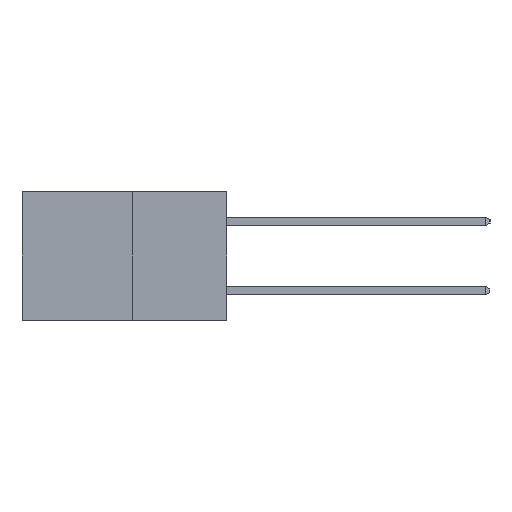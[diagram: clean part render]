
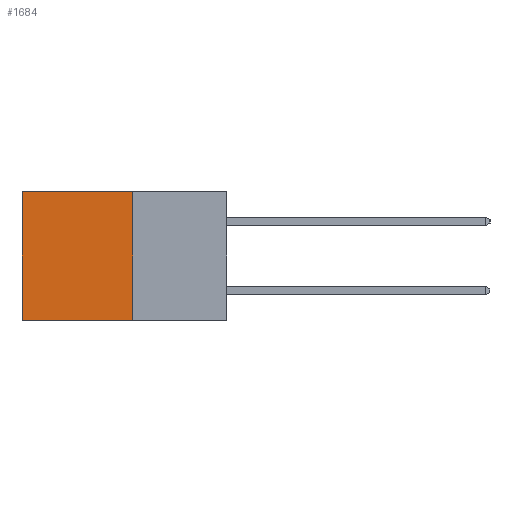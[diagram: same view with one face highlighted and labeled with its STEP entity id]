
A CAD part, left-side view. The second image highlights one B-rep face of the part: STEP entity #1684.
In plain terms, the highlighted planar face has unit normal (-1, 0, 0).
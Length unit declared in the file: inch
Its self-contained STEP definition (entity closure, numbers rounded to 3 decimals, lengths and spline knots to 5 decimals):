
#483 = VECTOR ( 'NONE', #691, 39.37008 ) ;
#499 = VERTEX_POINT ( 'NONE', #6705 ) ;
#691 = DIRECTION ( 'NONE',  ( 0., 1., 0. ) ) ;
#1018 = CARTESIAN_POINT ( 'NONE',  ( 0.277, 0.27, 0. ) ) ;
#1332 = EDGE_CURVE ( 'NONE', #8861, #1593, #4033, .T. ) ;
#1593 = VERTEX_POINT ( 'NONE', #8602 ) ;
#1684 = ADVANCED_FACE ( 'NONE', ( #2966 ), #6018, .F. ) ;
#2066 = VECTOR ( 'NONE', #5697, 39.37008 ) ;
#2381 = VECTOR ( 'NONE', #3738, 39.37008 ) ;
#2390 = LINE ( 'NONE', #8132, #8257 ) ;
#2966 = FACE_OUTER_BOUND ( 'NONE', #6873, .T. ) ;
#3132 = EDGE_CURVE ( 'NONE', #8741, #8861, #8332, .T. ) ;
#3738 = DIRECTION ( 'NONE',  ( 0., 0., -1. ) ) ;
#4033 = LINE ( 'NONE', #6846, #2066 ) ;
#4319 = CARTESIAN_POINT ( 'NONE',  ( 0.277, 0.27, -0.37 ) ) ;
#4415 = AXIS2_PLACEMENT_3D ( 'NONE', #4319, #5920, #5888 ) ;
#4494 = DIRECTION ( 'NONE',  ( 0., 1., 0. ) ) ;
#4719 = CARTESIAN_POINT ( 'NONE',  ( 0.277, 0.59, 0. ) ) ;
#5697 = DIRECTION ( 'NONE',  ( 0., 0., -1. ) ) ;
#5743 = ORIENTED_EDGE ( 'NONE', *, *, #3132, .T. ) ;
#5785 = ORIENTED_EDGE ( 'NONE', *, *, #7737, .F. ) ;
#5824 = ORIENTED_EDGE ( 'NONE', *, *, #7317, .F. ) ;
#5877 = ORIENTED_EDGE ( 'NONE', *, *, #1332, .T. ) ;
#5888 = DIRECTION ( 'NONE',  ( 0., 0., -1. ) ) ;
#5920 = DIRECTION ( 'NONE',  ( 1., 0., 0. ) ) ;
#6018 = PLANE ( 'NONE',  #4415 ) ;
#6705 = CARTESIAN_POINT ( 'NONE',  ( 0.277, 0.27, -0.37 ) ) ;
#6846 = CARTESIAN_POINT ( 'NONE',  ( 0.277, 0.59, -0.37 ) ) ;
#6873 = EDGE_LOOP ( 'NONE', ( #5877, #5824, #5785, #5743 ) ) ;
#7317 = EDGE_CURVE ( 'NONE', #499, #1593, #2390, .T. ) ;
#7400 = CARTESIAN_POINT ( 'NONE',  ( 0.277, 0.27, -0.37 ) ) ;
#7737 = EDGE_CURVE ( 'NONE', #8741, #499, #8692, .T. ) ;
#7858 = CARTESIAN_POINT ( 'NONE',  ( 0.277, 0.27, 0. ) ) ;
#8132 = CARTESIAN_POINT ( 'NONE',  ( 0.277, 0.27, -0.37 ) ) ;
#8257 = VECTOR ( 'NONE', #4494, 39.37008 ) ;
#8332 = LINE ( 'NONE', #1018, #483 ) ;
#8602 = CARTESIAN_POINT ( 'NONE',  ( 0.277, 0.59, -0.37 ) ) ;
#8692 = LINE ( 'NONE', #7400, #2381 ) ;
#8741 = VERTEX_POINT ( 'NONE', #7858 ) ;
#8861 = VERTEX_POINT ( 'NONE', #4719 ) ;
